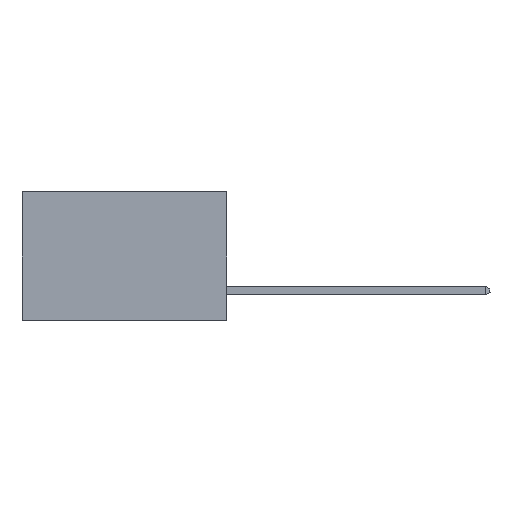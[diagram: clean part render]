
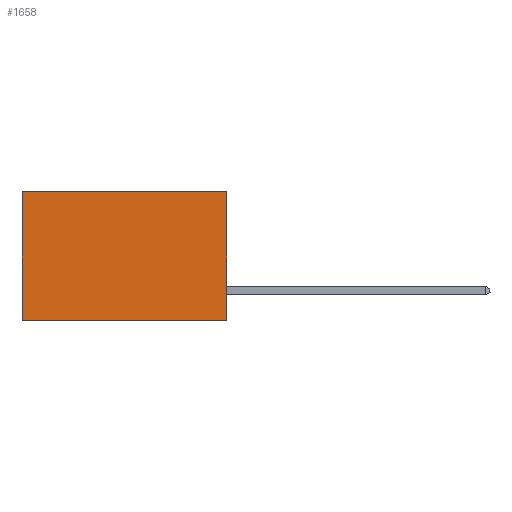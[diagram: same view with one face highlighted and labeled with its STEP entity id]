
A CAD part, left-side view. The second image highlights one B-rep face of the part: STEP entity #1658.
In plain terms, the highlighted planar face has unit normal (-1, 0, 0).
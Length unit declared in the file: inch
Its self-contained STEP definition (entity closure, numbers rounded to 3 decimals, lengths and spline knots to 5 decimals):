
#1038 = AXIS2_PLACEMENT_3D ( 'NONE', #14614, #25516, #7010 ) ;
#1658 = ADVANCED_FACE ( 'NONE', ( #19474 ), #22588, .F. ) ;
#1662 = EDGE_CURVE ( 'NONE', #1931, #21834, #6052, .T. ) ;
#1931 = VERTEX_POINT ( 'NONE', #6786 ) ;
#3326 = CARTESIAN_POINT ( 'NONE',  ( 0.277, 0., -0.37 ) ) ;
#3723 = DIRECTION ( 'NONE',  ( 0., 1., 0. ) ) ;
#5776 = EDGE_CURVE ( 'NONE', #21834, #13060, #13723, .T. ) ;
#6052 = LINE ( 'NONE', #18331, #6793 ) ;
#6786 = CARTESIAN_POINT ( 'NONE',  ( 0.277, 0., 0. ) ) ;
#6793 = VECTOR ( 'NONE', #10975, 39.37008 ) ;
#6975 = VERTEX_POINT ( 'NONE', #3326 ) ;
#7010 = DIRECTION ( 'NONE',  ( 0., 0., -1. ) ) ;
#7572 = VECTOR ( 'NONE', #18769, 39.37008 ) ;
#7607 = VECTOR ( 'NONE', #3723, 39.37008 ) ;
#9786 = CARTESIAN_POINT ( 'NONE',  ( 0.277, 0.59, -0.37 ) ) ;
#10413 = EDGE_LOOP ( 'NONE', ( #10589, #24892, #21988, #18016 ) ) ;
#10589 = ORIENTED_EDGE ( 'NONE', *, *, #5776, .T. ) ;
#10975 = DIRECTION ( 'NONE',  ( 0., 1., 0. ) ) ;
#11246 = LINE ( 'NONE', #17259, #23015 ) ;
#12650 = CARTESIAN_POINT ( 'NONE',  ( 0.277, 0.59, 0. ) ) ;
#13060 = VERTEX_POINT ( 'NONE', #28374 ) ;
#13723 = LINE ( 'NONE', #9786, #7572 ) ;
#14614 = CARTESIAN_POINT ( 'NONE',  ( 0.277, 0., -0.37 ) ) ;
#17259 = CARTESIAN_POINT ( 'NONE',  ( 0.277, 0., -0.37 ) ) ;
#18016 = ORIENTED_EDGE ( 'NONE', *, *, #1662, .T. ) ;
#18331 = CARTESIAN_POINT ( 'NONE',  ( 0.277, 0., 0. ) ) ;
#18769 = DIRECTION ( 'NONE',  ( 0., 0., -1. ) ) ;
#19474 = FACE_OUTER_BOUND ( 'NONE', #10413, .T. ) ;
#19777 = CARTESIAN_POINT ( 'NONE',  ( 0.277, 0., -0.37 ) ) ;
#19793 = LINE ( 'NONE', #19777, #7607 ) ;
#21793 = DIRECTION ( 'NONE',  ( 0., 0., -1. ) ) ;
#21834 = VERTEX_POINT ( 'NONE', #12650 ) ;
#21988 = ORIENTED_EDGE ( 'NONE', *, *, #23571, .F. ) ;
#22588 = PLANE ( 'NONE',  #1038 ) ;
#23015 = VECTOR ( 'NONE', #21793, 39.37008 ) ;
#23571 = EDGE_CURVE ( 'NONE', #1931, #6975, #11246, .T. ) ;
#24319 = EDGE_CURVE ( 'NONE', #6975, #13060, #19793, .T. ) ;
#24892 = ORIENTED_EDGE ( 'NONE', *, *, #24319, .F. ) ;
#25516 = DIRECTION ( 'NONE',  ( 1., 0., 0. ) ) ;
#28374 = CARTESIAN_POINT ( 'NONE',  ( 0.277, 0.59, -0.37 ) ) ;
